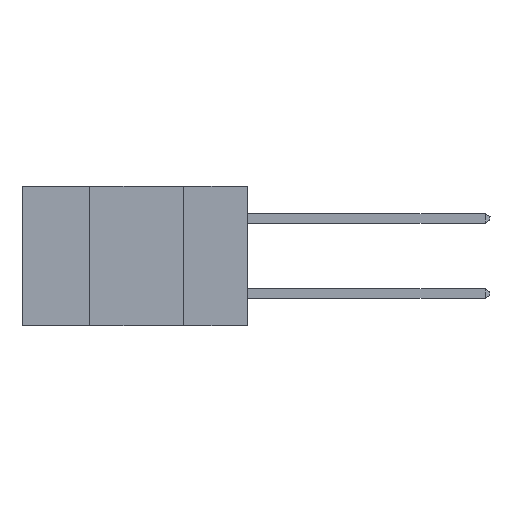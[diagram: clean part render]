
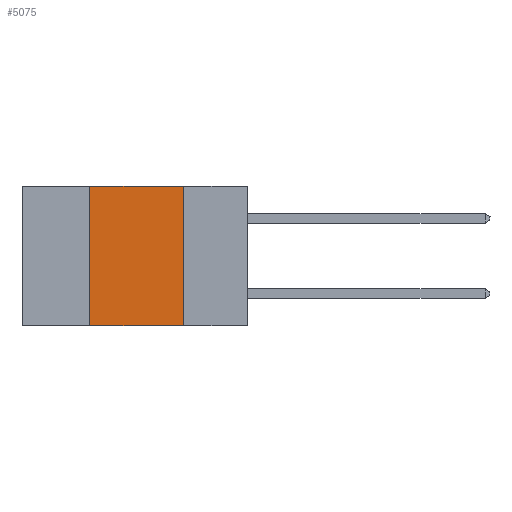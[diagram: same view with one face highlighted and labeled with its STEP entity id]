
A CAD part, left-side view. The second image highlights one B-rep face of the part: STEP entity #5075.
In plain terms, the highlighted planar face has unit normal (-1, 0, 0).
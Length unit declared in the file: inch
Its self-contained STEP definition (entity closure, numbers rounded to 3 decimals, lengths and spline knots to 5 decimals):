
#77 = VECTOR ( 'NONE', #15505, 39.37008 ) ;
#126 = ORIENTED_EDGE ( 'NONE', *, *, #6985, .F. ) ;
#609 = CARTESIAN_POINT ( 'NONE',  ( 0., 0.17, -0.37 ) ) ;
#671 = LINE ( 'NONE', #17195, #77 ) ;
#705 = EDGE_LOOP ( 'NONE', ( #7755, #126, #11837, #5008 ) ) ;
#1050 = DIRECTION ( 'NONE',  ( 0., 0., 1. ) ) ;
#1904 = CARTESIAN_POINT ( 'NONE',  ( 0., 0.17, 0. ) ) ;
#2029 = DIRECTION ( 'NONE',  ( 0., 0., -1. ) ) ;
#2530 = EDGE_CURVE ( 'NONE', #12551, #12581, #671, .T. ) ;
#3224 = DIRECTION ( 'NONE',  ( 0., -1., 0. ) ) ;
#3352 = VECTOR ( 'NONE', #3224, 39.37008 ) ;
#4317 = CARTESIAN_POINT ( 'NONE',  ( 0., 0.42, 0. ) ) ;
#4927 = CARTESIAN_POINT ( 'NONE',  ( 0., 0.17, -0.37 ) ) ;
#5008 = ORIENTED_EDGE ( 'NONE', *, *, #2530, .T. ) ;
#5075 = ADVANCED_FACE ( 'NONE', ( #9003 ), #18039, .F. ) ;
#5096 = LINE ( 'NONE', #609, #15234 ) ;
#5534 = LINE ( 'NONE', #8318, #12451 ) ;
#5812 = CARTESIAN_POINT ( 'NONE',  ( 0., 0.42, -0.37 ) ) ;
#6316 = LINE ( 'NONE', #15467, #3352 ) ;
#6985 = EDGE_CURVE ( 'NONE', #9182, #11788, #6316, .T. ) ;
#7408 = CARTESIAN_POINT ( 'NONE',  ( 0., 0.6, 0. ) ) ;
#7755 = ORIENTED_EDGE ( 'NONE', *, *, #16468, .F. ) ;
#8318 = CARTESIAN_POINT ( 'NONE',  ( 0., 0.42, -0.37 ) ) ;
#9003 = FACE_OUTER_BOUND ( 'NONE', #705, .T. ) ;
#9103 = DIRECTION ( 'NONE',  ( 1., 0., 0. ) ) ;
#9182 = VERTEX_POINT ( 'NONE', #4317 ) ;
#9709 = AXIS2_PLACEMENT_3D ( 'NONE', #7408, #9103, #13478 ) ;
#11788 = VERTEX_POINT ( 'NONE', #1904 ) ;
#11837 = ORIENTED_EDGE ( 'NONE', *, *, #17885, .F. ) ;
#12451 = VECTOR ( 'NONE', #1050, 39.37008 ) ;
#12551 = VERTEX_POINT ( 'NONE', #5812 ) ;
#12581 = VERTEX_POINT ( 'NONE', #4927 ) ;
#13478 = DIRECTION ( 'NONE',  ( 0., 0., -1. ) ) ;
#15234 = VECTOR ( 'NONE', #2029, 39.37008 ) ;
#15467 = CARTESIAN_POINT ( 'NONE',  ( 0., 0.6, 0. ) ) ;
#15505 = DIRECTION ( 'NONE',  ( 0., -1., 0. ) ) ;
#16468 = EDGE_CURVE ( 'NONE', #11788, #12581, #5096, .T. ) ;
#17195 = CARTESIAN_POINT ( 'NONE',  ( 0., 0.6, -0.37 ) ) ;
#17885 = EDGE_CURVE ( 'NONE', #12551, #9182, #5534, .T. ) ;
#18039 = PLANE ( 'NONE',  #9709 ) ;
